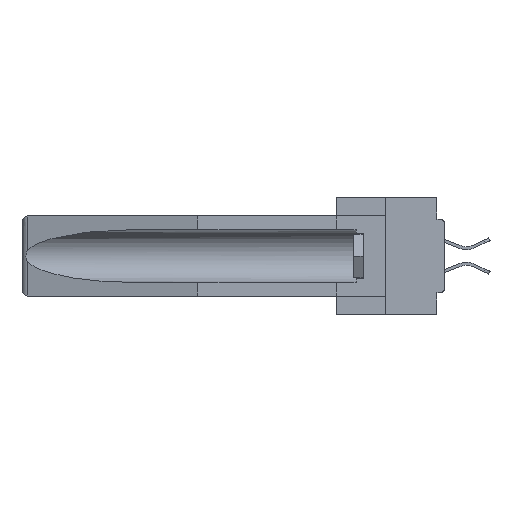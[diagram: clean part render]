
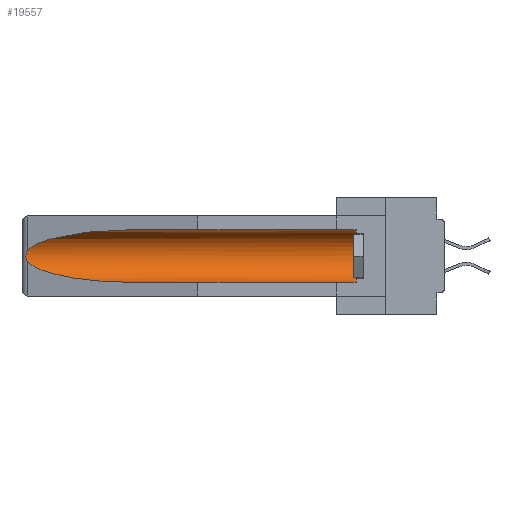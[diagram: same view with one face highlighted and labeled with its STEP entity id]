
A CAD part, left-side view. The second image highlights one B-rep face of the part: STEP entity #19557.
In plain terms, the highlighted cylindrical face has radius 2.857 mm (diameter 5.715 mm), a partial arc.
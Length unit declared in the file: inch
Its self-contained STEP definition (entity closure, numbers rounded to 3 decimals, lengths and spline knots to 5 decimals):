
#1457 = VERTEX_POINT ( 'NONE', #39175 ) ;
#3900 = CARTESIAN_POINT ( 'NONE',  ( 0.155, -0.30754, -0.1715 ) ) ;
#4340 = DIRECTION ( 'NONE',  ( 0., 1., 0. ) ) ;
#5377 = CARTESIAN_POINT ( 'NONE',  ( 0.21114, 1.30732, -0.284 ) ) ;
#5808 = CIRCLE ( 'NONE', #15999, 0.1125 ) ;
#6276 = CARTESIAN_POINT ( 'NONE',  ( 0.26537, 1.52718, -0.19328 ) ) ;
#8898 = CARTESIAN_POINT ( 'NONE',  ( 0.26597, 1.5296, -0.19026 ) ) ;
#9362 = VECTOR ( 'NONE', #11805, 39.37008 ) ;
#9425 = VERTEX_POINT ( 'NONE', #25045 ) ;
#10246 = CARTESIAN_POINT ( 'NONE',  ( 0.155, 1.07973, -0.059 ) ) ;
#10322 = DIRECTION ( 'NONE',  ( 0., -1., 0. ) ) ;
#10840 = CARTESIAN_POINT ( 'NONE',  ( 0.155, -0.30754, -0.059 ) ) ;
#11391 = ORIENTED_EDGE ( 'NONE', *, *, #29220, .T. ) ;
#11805 = DIRECTION ( 'NONE',  ( 0., 1., 0. ) ) ;
#11837 = EDGE_CURVE ( 'NONE', #1457, #15641, #25406, .T. ) ;
#12344 = CARTESIAN_POINT ( 'NONE',  ( 0.26537, 1.52718, -0.14972 ) ) ;
#13191 = VERTEX_POINT ( 'NONE', #19738 ) ;
#14402 = EDGE_CURVE ( 'NONE', #15641, #9425, #27325, .T. ) ;
#14417 = CARTESIAN_POINT ( 'NONE',  ( 0.2673, 1.5327, -0.16383 ) ) ;
#14523 = CARTESIAN_POINT ( 'NONE',  ( 0.2673, 1.53269, -0.17917 ) ) ;
#14688 = EDGE_LOOP ( 'NONE', ( #34920, #30180, #40545, #39317, #11391, #21681 ) ) ;
#15277 = CARTESIAN_POINT ( 'NONE',  ( 0.26537, 1.52718, -0.19328 ) ) ;
#15285 = EDGE_CURVE ( 'NONE', #9425, #13191, #30595, .T. ) ;
#15641 = VERTEX_POINT ( 'NONE', #41188 ) ;
#15999 = AXIS2_PLACEMENT_3D ( 'NONE', #43352, #10322, #33085 ) ;
#17575 = CYLINDRICAL_SURFACE ( 'NONE', #19679, 0.1125 ) ;
#18228 = EDGE_CURVE ( 'NONE', #30987, #13191, #20281, .T. ) ;
#19557 = ADVANCED_FACE ( 'NONE', ( #27487 ), #17575, .F. ) ;
#19679 = AXIS2_PLACEMENT_3D ( 'NONE', #3900, #4340, #27678 ) ;
#19738 = CARTESIAN_POINT ( 'NONE',  ( 0.155, 1.07973, -0.284 ) ) ;
#20281 = LINE ( 'NONE', #37810, #39684 ) ;
#20283 = CARTESIAN_POINT ( 'NONE',  ( 0.25451, 1.48313, -0.09465 ) ) ;
#21519 = CARTESIAN_POINT ( 'NONE',  ( 0.26597, 1.52961, -0.15275 ) ) ;
#21606 = VERTEX_POINT ( 'NONE', #40973 ) ;
#21681 = ORIENTED_EDGE ( 'NONE', *, *, #30151, .T. ) ;
#23634 = CARTESIAN_POINT ( 'NONE',  ( 0.26537, 1.52718, -0.14972 ) ) ;
#23919 = CARTESIAN_POINT ( 'NONE',  ( 0.26654, 1.53092, -0.15636 ) ) ;
#25045 = CARTESIAN_POINT ( 'NONE',  ( 0.26537, 1.52718, -0.19328 ) ) ;
#25185 = CARTESIAN_POINT ( 'NONE',  ( 0.25451, 1.48313, -0.24835 ) ) ;
#25406 =( BOUNDED_CURVE ( )  B_SPLINE_CURVE ( 3, ( #10246, #40377, #20283, #23634 ),
 .UNSPECIFIED., .F., .T. ) 
 B_SPLINE_CURVE_WITH_KNOTS ( ( 4, 4 ),
 ( 4.71239, 6.08839 ),
 .UNSPECIFIED. ) 
 CURVE ( )  GEOMETRIC_REPRESENTATION_ITEM ( )  RATIONAL_B_SPLINE_CURVE ( ( 1., 0.848, 0.848, 1. ) ) 
 REPRESENTATION_ITEM ( '' )  );
#27325 = B_SPLINE_CURVE_WITH_KNOTS ( 'NONE', 3,
 ( #12344, #21519, #23919, #14417, #42934, #29863, #14523, #28843, #8898, #6276 ),
 .UNSPECIFIED., .F., .F.,
 ( 4, 2, 2, 2, 4 ),
 ( 0., 0.00029, 0.00058, 0.00087, 0.00117 ),
 .UNSPECIFIED. ) ;
#27487 = FACE_OUTER_BOUND ( 'NONE', #14688, .T. ) ;
#27678 = DIRECTION ( 'NONE',  ( 0., 0., 1. ) ) ;
#28843 = CARTESIAN_POINT ( 'NONE',  ( 0.26655, 1.53094, -0.18657 ) ) ;
#29220 = EDGE_CURVE ( 'NONE', #30987, #21606, #5808, .T. ) ;
#29863 = CARTESIAN_POINT ( 'NONE',  ( 0.2675, 1.53308, -0.17534 ) ) ;
#30151 = EDGE_CURVE ( 'NONE', #21606, #1457, #38161, .T. ) ;
#30180 = ORIENTED_EDGE ( 'NONE', *, *, #14402, .T. ) ;
#30595 =( BOUNDED_CURVE ( )  B_SPLINE_CURVE ( 3, ( #15277, #25185, #5377, #42246 ),
 .UNSPECIFIED., .F., .F. ) 
 B_SPLINE_CURVE_WITH_KNOTS ( ( 4, 4 ),
 ( 0.1948, 1.5708 ),
 .UNSPECIFIED. ) 
 CURVE ( )  GEOMETRIC_REPRESENTATION_ITEM ( )  RATIONAL_B_SPLINE_CURVE ( ( 1., 0.848, 0.848, 1. ) ) 
 REPRESENTATION_ITEM ( '' )  );
#30987 = VERTEX_POINT ( 'NONE', #41502 ) ;
#31364 = DIRECTION ( 'NONE',  ( 0., 1., 0. ) ) ;
#33085 = DIRECTION ( 'NONE',  ( 0., 0., 1. ) ) ;
#34920 = ORIENTED_EDGE ( 'NONE', *, *, #11837, .T. ) ;
#37810 = CARTESIAN_POINT ( 'NONE',  ( 0.155, -0.30754, -0.284 ) ) ;
#38161 = LINE ( 'NONE', #10840, #9362 ) ;
#39175 = CARTESIAN_POINT ( 'NONE',  ( 0.155, 1.07973, -0.059 ) ) ;
#39317 = ORIENTED_EDGE ( 'NONE', *, *, #18228, .F. ) ;
#39684 = VECTOR ( 'NONE', #31364, 39.37008 ) ;
#40377 = CARTESIAN_POINT ( 'NONE',  ( 0.21114, 1.30732, -0.059 ) ) ;
#40545 = ORIENTED_EDGE ( 'NONE', *, *, #15285, .T. ) ;
#40973 = CARTESIAN_POINT ( 'NONE',  ( 0.155, 0.126, -0.059 ) ) ;
#41188 = CARTESIAN_POINT ( 'NONE',  ( 0.26537, 1.52718, -0.14972 ) ) ;
#41502 = CARTESIAN_POINT ( 'NONE',  ( 0.155, 0.126, -0.284 ) ) ;
#42246 = CARTESIAN_POINT ( 'NONE',  ( 0.155, 1.07973, -0.284 ) ) ;
#42934 = CARTESIAN_POINT ( 'NONE',  ( 0.2675, 1.53308, -0.16763 ) ) ;
#43352 = CARTESIAN_POINT ( 'NONE',  ( 0.155, 0.126, -0.1715 ) ) ;
